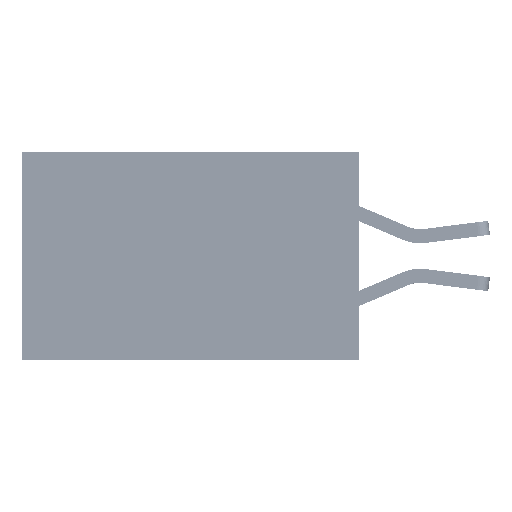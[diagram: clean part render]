
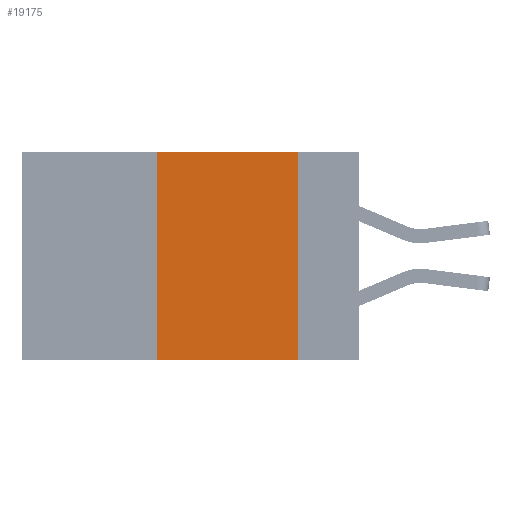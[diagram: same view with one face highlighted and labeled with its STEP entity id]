
A CAD part, left-side view. The second image highlights one B-rep face of the part: STEP entity #19175.
In plain terms, the highlighted planar face has unit normal (-1, 0, 0).
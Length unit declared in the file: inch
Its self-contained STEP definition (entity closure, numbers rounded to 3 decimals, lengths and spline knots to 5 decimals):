
#501 = ORIENTED_EDGE ( 'NONE', *, *, #8715, .F. ) ;
#696 = ORIENTED_EDGE ( 'NONE', *, *, #3141, .F. ) ;
#749 = DIRECTION ( 'NONE',  ( 0., -1., 0. ) ) ;
#1843 = VERTEX_POINT ( 'NONE', #29925 ) ;
#1925 = DIRECTION ( 'NONE',  ( 1., 0., 0. ) ) ;
#2396 = CARTESIAN_POINT ( 'NONE',  ( 0., 0.6, 0. ) ) ;
#3141 = EDGE_CURVE ( 'NONE', #32936, #1843, #15468, .T. ) ;
#7135 = VECTOR ( 'NONE', #42734, 39.37008 ) ;
#8715 = EDGE_CURVE ( 'NONE', #1843, #33846, #21011, .T. ) ;
#9536 = CARTESIAN_POINT ( 'NONE',  ( 0., 0.36, 0. ) ) ;
#9581 = VECTOR ( 'NONE', #749, 39.37008 ) ;
#10686 = VERTEX_POINT ( 'NONE', #16207 ) ;
#11711 = AXIS2_PLACEMENT_3D ( 'NONE', #2396, #1925, #31559 ) ;
#15468 = LINE ( 'NONE', #37752, #9581 ) ;
#15660 = VECTOR ( 'NONE', #39284, 39.37008 ) ;
#16207 = CARTESIAN_POINT ( 'NONE',  ( 0., 0.36, -0.37 ) ) ;
#19175 = ADVANCED_FACE ( 'NONE', ( #30639 ), #34419, .F. ) ;
#19343 = EDGE_CURVE ( 'NONE', #10686, #33846, #28490, .T. ) ;
#20954 = EDGE_LOOP ( 'NONE', ( #501, #696, #45085, #22991 ) ) ;
#21011 = LINE ( 'NONE', #32152, #15660 ) ;
#22991 = ORIENTED_EDGE ( 'NONE', *, *, #19343, .T. ) ;
#25467 = DIRECTION ( 'NONE',  ( 0., 0., 1. ) ) ;
#26551 = EDGE_CURVE ( 'NONE', #10686, #32936, #39239, .T. ) ;
#27694 = CARTESIAN_POINT ( 'NONE',  ( 0., 0.11, -0.37 ) ) ;
#28490 = LINE ( 'NONE', #43433, #7135 ) ;
#29925 = CARTESIAN_POINT ( 'NONE',  ( 0., 0.11, 0. ) ) ;
#30639 = FACE_OUTER_BOUND ( 'NONE', #20954, .T. ) ;
#31559 = DIRECTION ( 'NONE',  ( 0., 0., -1. ) ) ;
#32109 = CARTESIAN_POINT ( 'NONE',  ( 0., 0.36, 0. ) ) ;
#32152 = CARTESIAN_POINT ( 'NONE',  ( 0., 0.11, 0. ) ) ;
#32936 = VERTEX_POINT ( 'NONE', #9536 ) ;
#33846 = VERTEX_POINT ( 'NONE', #27694 ) ;
#34419 = PLANE ( 'NONE',  #11711 ) ;
#35264 = VECTOR ( 'NONE', #25467, 39.37008 ) ;
#37752 = CARTESIAN_POINT ( 'NONE',  ( 0., 0.6, 0. ) ) ;
#39239 = LINE ( 'NONE', #32109, #35264 ) ;
#39284 = DIRECTION ( 'NONE',  ( 0., 0., -1. ) ) ;
#42734 = DIRECTION ( 'NONE',  ( 0., -1., 0. ) ) ;
#43433 = CARTESIAN_POINT ( 'NONE',  ( 0., 0.6, -0.37 ) ) ;
#45085 = ORIENTED_EDGE ( 'NONE', *, *, #26551, .F. ) ;
